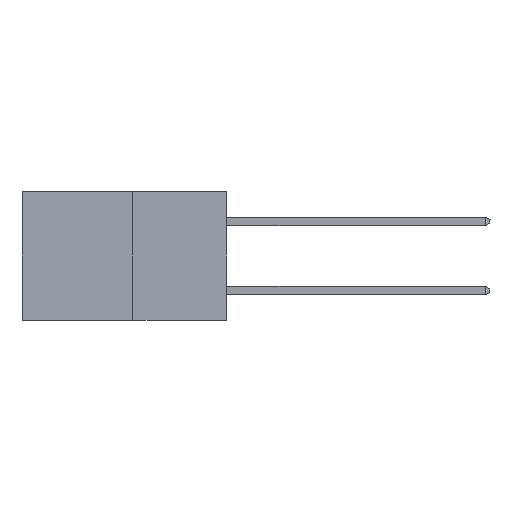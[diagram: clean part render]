
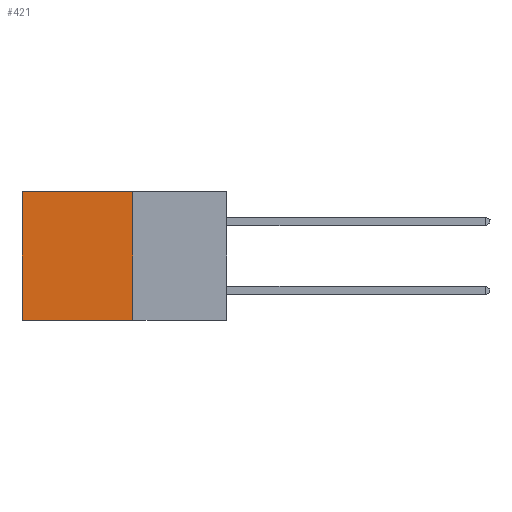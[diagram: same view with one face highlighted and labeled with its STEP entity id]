
A CAD part, left-side view. The second image highlights one B-rep face of the part: STEP entity #421.
In plain terms, the highlighted planar face has unit normal (-1, 0, 0).
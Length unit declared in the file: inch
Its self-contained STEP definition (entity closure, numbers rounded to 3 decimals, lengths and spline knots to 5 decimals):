
#421 = ADVANCED_FACE ( 'NONE', ( #9198 ), #6792, .F. ) ;
#535 = LINE ( 'NONE', #4438, #2206 ) ;
#914 = LINE ( 'NONE', #5032, #4852 ) ;
#1271 = EDGE_CURVE ( 'NONE', #5485, #6805, #535, .T. ) ;
#1278 = LINE ( 'NONE', #3116, #5181 ) ;
#1466 = EDGE_CURVE ( 'NONE', #5485, #2373, #914, .T. ) ;
#2012 = DIRECTION ( 'NONE',  ( 1., 0., 0. ) ) ;
#2126 = CARTESIAN_POINT ( 'NONE',  ( 0.277, 0.27, 0. ) ) ;
#2206 = VECTOR ( 'NONE', #5696, 39.37008 ) ;
#2373 = VERTEX_POINT ( 'NONE', #8884 ) ;
#2422 = ORIENTED_EDGE ( 'NONE', *, *, #1466, .F. ) ;
#2489 = DIRECTION ( 'NONE',  ( 0., 0., -1. ) ) ;
#2535 = VERTEX_POINT ( 'NONE', #5088 ) ;
#3116 = CARTESIAN_POINT ( 'NONE',  ( 0.277, 0.27, -0.37 ) ) ;
#3926 = DIRECTION ( 'NONE',  ( 0., 1., 0. ) ) ;
#4009 = CARTESIAN_POINT ( 'NONE',  ( 0.277, 0.59, 0. ) ) ;
#4158 = DIRECTION ( 'NONE',  ( 0., 0., -1. ) ) ;
#4177 = EDGE_CURVE ( 'NONE', #2373, #2535, #1278, .T. ) ;
#4235 = AXIS2_PLACEMENT_3D ( 'NONE', #5876, #2012, #4158 ) ;
#4438 = CARTESIAN_POINT ( 'NONE',  ( 0.277, 0.27, 0. ) ) ;
#4568 = ORIENTED_EDGE ( 'NONE', *, *, #1271, .T. ) ;
#4852 = VECTOR ( 'NONE', #5124, 39.37008 ) ;
#5032 = CARTESIAN_POINT ( 'NONE',  ( 0.277, 0.27, -0.37 ) ) ;
#5088 = CARTESIAN_POINT ( 'NONE',  ( 0.277, 0.59, -0.37 ) ) ;
#5124 = DIRECTION ( 'NONE',  ( 0., 0., -1. ) ) ;
#5181 = VECTOR ( 'NONE', #3926, 39.37008 ) ;
#5369 = VECTOR ( 'NONE', #2489, 39.37008 ) ;
#5485 = VERTEX_POINT ( 'NONE', #2126 ) ;
#5696 = DIRECTION ( 'NONE',  ( 0., 1., 0. ) ) ;
#5876 = CARTESIAN_POINT ( 'NONE',  ( 0.277, 0.27, -0.37 ) ) ;
#6792 = PLANE ( 'NONE',  #4235 ) ;
#6805 = VERTEX_POINT ( 'NONE', #4009 ) ;
#6902 = ORIENTED_EDGE ( 'NONE', *, *, #9251, .T. ) ;
#7310 = LINE ( 'NONE', #7710, #5369 ) ;
#7530 = ORIENTED_EDGE ( 'NONE', *, *, #4177, .F. ) ;
#7710 = CARTESIAN_POINT ( 'NONE',  ( 0.277, 0.59, -0.37 ) ) ;
#7916 = EDGE_LOOP ( 'NONE', ( #6902, #7530, #2422, #4568 ) ) ;
#8884 = CARTESIAN_POINT ( 'NONE',  ( 0.277, 0.27, -0.37 ) ) ;
#9198 = FACE_OUTER_BOUND ( 'NONE', #7916, .T. ) ;
#9251 = EDGE_CURVE ( 'NONE', #6805, #2535, #7310, .T. ) ;
